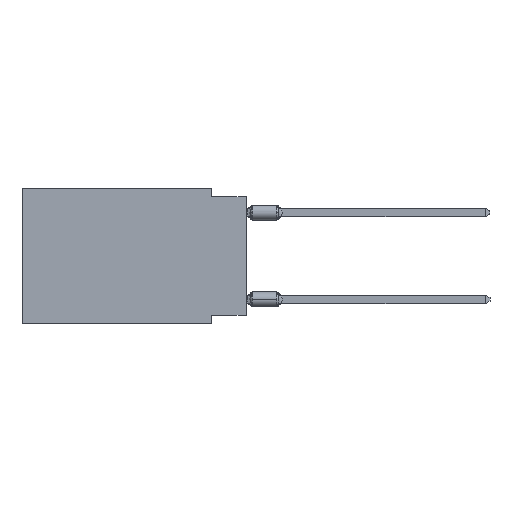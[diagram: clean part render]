
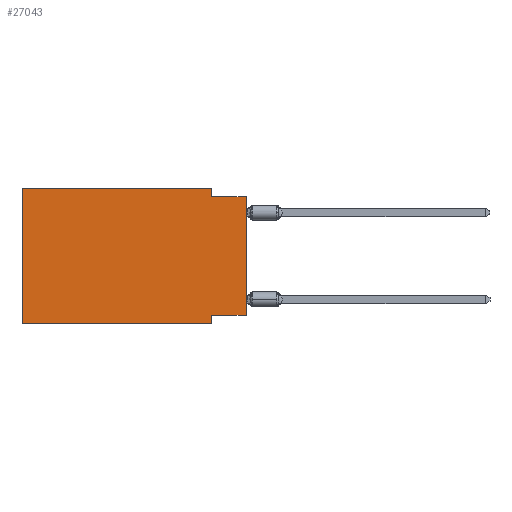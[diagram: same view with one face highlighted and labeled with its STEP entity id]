
A CAD part, left-side view. The second image highlights one B-rep face of the part: STEP entity #27043.
In plain terms, the highlighted planar face has unit normal (-1, 0, 0).
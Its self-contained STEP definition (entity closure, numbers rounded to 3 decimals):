
#677 = VERTEX_POINT ( 'NONE', #22957 ) ;
#732 = VECTOR ( 'NONE', #2998, 1000. ) ;
#1936 = CARTESIAN_POINT ( 'NONE',  ( 0., 0., 0. ) ) ;
#2090 = LINE ( 'NONE', #7358, #13079 ) ;
#2278 = EDGE_CURVE ( 'NONE', #19261, #30344, #25369, .T. ) ;
#2796 = CARTESIAN_POINT ( 'NONE',  ( 0., 16.383, 0. ) ) ;
#2998 = DIRECTION ( 'NONE',  ( 0., 0., -1. ) ) ;
#3162 = CARTESIAN_POINT ( 'NONE',  ( 0., 16.383, 0. ) ) ;
#3424 = ORIENTED_EDGE ( 'NONE', *, *, #16517, .T. ) ;
#3425 = VECTOR ( 'NONE', #22902, 1000. ) ;
#3427 = VERTEX_POINT ( 'NONE', #8222 ) ;
#3645 = PLANE ( 'NONE',  #20359 ) ;
#3782 = CARTESIAN_POINT ( 'NONE',  ( 0., 16.383, 0. ) ) ;
#4733 = EDGE_CURVE ( 'NONE', #30344, #3427, #8119, .T. ) ;
#5474 = LINE ( 'NONE', #25423, #732 ) ;
#5590 = LINE ( 'NONE', #10707, #7756 ) ;
#5647 = EDGE_CURVE ( 'NONE', #3427, #12586, #27618, .T. ) ;
#5744 = ORIENTED_EDGE ( 'NONE', *, *, #18744, .F. ) ;
#5927 = ORIENTED_EDGE ( 'NONE', *, *, #5647, .F. ) ;
#6281 = EDGE_CURVE ( 'NONE', #9988, #23043, #5474, .T. ) ;
#7358 = CARTESIAN_POINT ( 'NONE',  ( 0., 0., -0.635 ) ) ;
#7504 = DIRECTION ( 'NONE',  ( 0., 0., -1. ) ) ;
#7724 = CARTESIAN_POINT ( 'NONE',  ( 0., 2.54, -9.906 ) ) ;
#7756 = VECTOR ( 'NONE', #26357, 1000. ) ;
#8119 = LINE ( 'NONE', #3782, #29008 ) ;
#8222 = CARTESIAN_POINT ( 'NONE',  ( 0., 2.54, 0. ) ) ;
#8587 = VECTOR ( 'NONE', #32118, 1000. ) ;
#9438 = LINE ( 'NONE', #14529, #13724 ) ;
#9988 = VERTEX_POINT ( 'NONE', #22606 ) ;
#10707 = CARTESIAN_POINT ( 'NONE',  ( 0., 0., -9.271 ) ) ;
#11279 = ORIENTED_EDGE ( 'NONE', *, *, #14386, .T. ) ;
#12311 = LINE ( 'NONE', #1936, #8587 ) ;
#12325 = VERTEX_POINT ( 'NONE', #16396 ) ;
#12586 = VERTEX_POINT ( 'NONE', #13240 ) ;
#13049 = DIRECTION ( 'NONE',  ( 0., 0., -1. ) ) ;
#13079 = VECTOR ( 'NONE', #29765, 1000. ) ;
#13240 = CARTESIAN_POINT ( 'NONE',  ( 0., 2.54, -0.635 ) ) ;
#13289 = ORIENTED_EDGE ( 'NONE', *, *, #23417, .F. ) ;
#13628 = ORIENTED_EDGE ( 'NONE', *, *, #4733, .F. ) ;
#13724 = VECTOR ( 'NONE', #24752, 1000. ) ;
#14386 = EDGE_CURVE ( 'NONE', #19261, #23043, #9438, .T. ) ;
#14456 = CARTESIAN_POINT ( 'NONE',  ( 0., 16.383, 0. ) ) ;
#14529 = CARTESIAN_POINT ( 'NONE',  ( 0., 16.383, -9.906 ) ) ;
#16396 = CARTESIAN_POINT ( 'NONE',  ( 0., 0., -0.635 ) ) ;
#16467 = DIRECTION ( 'NONE',  ( 0., -1., 0. ) ) ;
#16517 = EDGE_CURVE ( 'NONE', #677, #12325, #12311, .T. ) ;
#18744 = EDGE_CURVE ( 'NONE', #677, #9988, #5590, .T. ) ;
#19261 = VERTEX_POINT ( 'NONE', #21197 ) ;
#20359 = AXIS2_PLACEMENT_3D ( 'NONE', #3162, #28530, #13049 ) ;
#21197 = CARTESIAN_POINT ( 'NONE',  ( 0., 16.383, -9.906 ) ) ;
#22124 = VECTOR ( 'NONE', #7504, 1000. ) ;
#22606 = CARTESIAN_POINT ( 'NONE',  ( 0., 2.54, -9.271 ) ) ;
#22687 = ORIENTED_EDGE ( 'NONE', *, *, #2278, .F. ) ;
#22902 = DIRECTION ( 'NONE',  ( 0., 0., 1. ) ) ;
#22957 = CARTESIAN_POINT ( 'NONE',  ( 0., 0., -9.271 ) ) ;
#23043 = VERTEX_POINT ( 'NONE', #7724 ) ;
#23417 = EDGE_CURVE ( 'NONE', #12586, #12325, #2090, .T. ) ;
#23934 = EDGE_LOOP ( 'NONE', ( #3424, #13289, #5927, #13628, #22687, #11279, #31324, #5744 ) ) ;
#24752 = DIRECTION ( 'NONE',  ( 0., -1., 0. ) ) ;
#25369 = LINE ( 'NONE', #2796, #3425 ) ;
#25423 = CARTESIAN_POINT ( 'NONE',  ( 0., 2.54, -9.906 ) ) ;
#25892 = FACE_OUTER_BOUND ( 'NONE', #23934, .T. ) ;
#26357 = DIRECTION ( 'NONE',  ( 0., 1., 0. ) ) ;
#27043 = ADVANCED_FACE ( 'NONE', ( #25892 ), #3645, .F. ) ;
#27618 = LINE ( 'NONE', #32400, #22124 ) ;
#28530 = DIRECTION ( 'NONE',  ( 1., 0., 0. ) ) ;
#29008 = VECTOR ( 'NONE', #16467, 1000. ) ;
#29765 = DIRECTION ( 'NONE',  ( 0., -1., 0. ) ) ;
#30344 = VERTEX_POINT ( 'NONE', #14456 ) ;
#31324 = ORIENTED_EDGE ( 'NONE', *, *, #6281, .F. ) ;
#32118 = DIRECTION ( 'NONE',  ( 0., 0., 1. ) ) ;
#32400 = CARTESIAN_POINT ( 'NONE',  ( 0., 2.54, 0. ) ) ;
